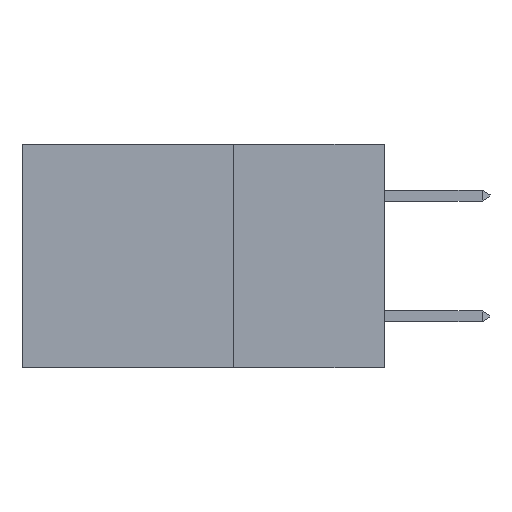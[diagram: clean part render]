
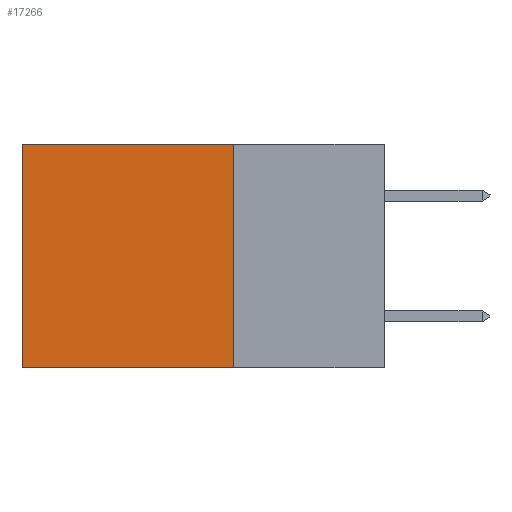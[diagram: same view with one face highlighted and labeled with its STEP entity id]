
A CAD part, left-side view. The second image highlights one B-rep face of the part: STEP entity #17266.
In plain terms, the highlighted planar face has unit normal (-1, 0, 0).
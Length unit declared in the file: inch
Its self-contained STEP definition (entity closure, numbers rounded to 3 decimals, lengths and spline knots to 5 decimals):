
#1327 = DIRECTION ( 'NONE',  ( 0., 1., 0. ) ) ;
#1762 = EDGE_CURVE ( 'NONE', #16924, #25381, #35379, .T. ) ;
#1888 = DIRECTION ( 'NONE',  ( 0., 0., -1. ) ) ;
#2627 = CARTESIAN_POINT ( 'NONE',  ( 0.2875, 0.25, 0. ) ) ;
#4221 = EDGE_CURVE ( 'NONE', #23171, #25381, #36055, .T. ) ;
#4296 = CARTESIAN_POINT ( 'NONE',  ( 0.2875, 0.6, 0. ) ) ;
#6727 = VERTEX_POINT ( 'NONE', #34999 ) ;
#7465 = ORIENTED_EDGE ( 'NONE', *, *, #1762, .F. ) ;
#7797 = EDGE_CURVE ( 'NONE', #6727, #23171, #15272, .T. ) ;
#8328 = ORIENTED_EDGE ( 'NONE', *, *, #7797, .T. ) ;
#8384 = DIRECTION ( 'NONE',  ( 0., 0., -1. ) ) ;
#12708 = CARTESIAN_POINT ( 'NONE',  ( 0.2875, 0.25, 0. ) ) ;
#13732 = CARTESIAN_POINT ( 'NONE',  ( 0.2875, 0.25, -0.37 ) ) ;
#13771 = DIRECTION ( 'NONE',  ( 1., 0., 0. ) ) ;
#15183 = LINE ( 'NONE', #19627, #25451 ) ;
#15272 = LINE ( 'NONE', #12708, #34948 ) ;
#16466 = AXIS2_PLACEMENT_3D ( 'NONE', #2627, #13771, #8384 ) ;
#16924 = VERTEX_POINT ( 'NONE', #17012 ) ;
#17012 = CARTESIAN_POINT ( 'NONE',  ( 0.2875, 0.25, -0.37 ) ) ;
#17266 = ADVANCED_FACE ( 'NONE', ( #28918 ), #25110, .F. ) ;
#18237 = CARTESIAN_POINT ( 'NONE',  ( 0.2875, 0.6, -0.37 ) ) ;
#19627 = CARTESIAN_POINT ( 'NONE',  ( 0.2875, 0.25, 0. ) ) ;
#19956 = EDGE_CURVE ( 'NONE', #6727, #16924, #15183, .T. ) ;
#21024 = EDGE_LOOP ( 'NONE', ( #29207, #7465, #33580, #8328 ) ) ;
#23171 = VERTEX_POINT ( 'NONE', #4296 ) ;
#25110 = PLANE ( 'NONE',  #16466 ) ;
#25381 = VERTEX_POINT ( 'NONE', #18237 ) ;
#25451 = VECTOR ( 'NONE', #36376, 39.37008 ) ;
#28918 = FACE_OUTER_BOUND ( 'NONE', #21024, .T. ) ;
#29207 = ORIENTED_EDGE ( 'NONE', *, *, #4221, .T. ) ;
#31067 = DIRECTION ( 'NONE',  ( 0., 1., 0. ) ) ;
#32877 = CARTESIAN_POINT ( 'NONE',  ( 0.2875, 0.6, 0. ) ) ;
#33366 = VECTOR ( 'NONE', #1888, 39.37008 ) ;
#33580 = ORIENTED_EDGE ( 'NONE', *, *, #19956, .F. ) ;
#34948 = VECTOR ( 'NONE', #1327, 39.37008 ) ;
#34999 = CARTESIAN_POINT ( 'NONE',  ( 0.2875, 0.25, 0. ) ) ;
#35379 = LINE ( 'NONE', #13732, #35806 ) ;
#35806 = VECTOR ( 'NONE', #31067, 39.37008 ) ;
#36055 = LINE ( 'NONE', #32877, #33366 ) ;
#36376 = DIRECTION ( 'NONE',  ( 0., 0., -1. ) ) ;
